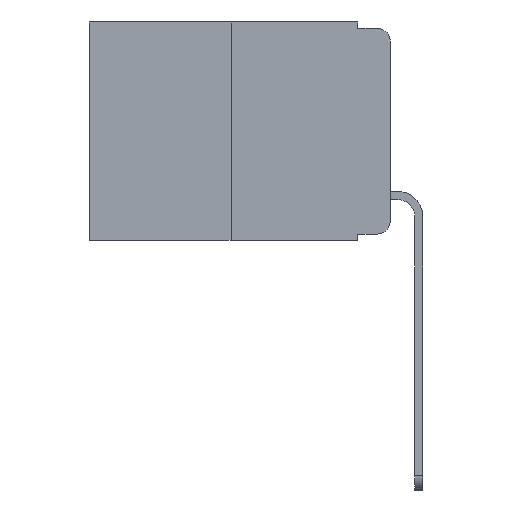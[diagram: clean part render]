
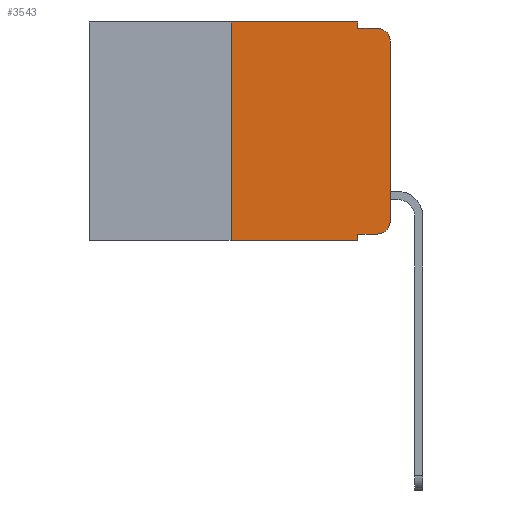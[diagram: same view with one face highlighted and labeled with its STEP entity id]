
A CAD part, left-side view. The second image highlights one B-rep face of the part: STEP entity #3543.
In plain terms, the highlighted planar face has unit normal (-1, 0, 0).
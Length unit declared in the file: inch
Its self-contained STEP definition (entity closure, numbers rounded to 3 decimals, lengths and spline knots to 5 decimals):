
#118 = VECTOR ( 'NONE', #10049, 39.37008 ) ;
#206 = EDGE_CURVE ( 'NONE', #10461, #6920, #1319, .T. ) ;
#211 = ORIENTED_EDGE ( 'NONE', *, *, #8891, .F. ) ;
#290 = DIRECTION ( 'NONE',  ( 0., 0., -1. ) ) ;
#351 = AXIS2_PLACEMENT_3D ( 'NONE', #6485, #12256, #6536 ) ;
#1319 = LINE ( 'NONE', #1860, #9890 ) ;
#1368 = DIRECTION ( 'NONE',  ( 0., 0., -1. ) ) ;
#1842 = CARTESIAN_POINT ( 'NONE',  ( 0., 0., -0.03 ) ) ;
#1860 = CARTESIAN_POINT ( 'NONE',  ( 0., 0.473, 0. ) ) ;
#2236 = LINE ( 'NONE', #7683, #118 ) ;
#2592 = CARTESIAN_POINT ( 'NONE',  ( 0., 0., -0.313 ) ) ;
#2613 = CARTESIAN_POINT ( 'NONE',  ( 0., 0.02, -0.01 ) ) ;
#2663 = DIRECTION ( 'NONE',  ( 0., -1., 0. ) ) ;
#2763 = CARTESIAN_POINT ( 'NONE',  ( 0., 0.051, -0.01 ) ) ;
#3039 = DIRECTION ( 'NONE',  ( 0., 0., -1. ) ) ;
#3083 = CARTESIAN_POINT ( 'NONE',  ( 0., 0.051, -0.333 ) ) ;
#3187 = ORIENTED_EDGE ( 'NONE', *, *, #206, .F. ) ;
#3426 = VERTEX_POINT ( 'NONE', #9632 ) ;
#3506 = CIRCLE ( 'NONE', #7807, 0.02 ) ;
#3536 = LINE ( 'NONE', #11084, #14057 ) ;
#3543 = ADVANCED_FACE ( 'NONE', ( #4294 ), #5477, .F. ) ;
#3706 = EDGE_CURVE ( 'NONE', #3426, #8450, #5513, .T. ) ;
#4294 = FACE_OUTER_BOUND ( 'NONE', #13301, .T. ) ;
#4432 = VECTOR ( 'NONE', #2663, 39.37008 ) ;
#4646 = CARTESIAN_POINT ( 'NONE',  ( 0., 0.051, 0. ) ) ;
#4722 = EDGE_CURVE ( 'NONE', #13877, #8409, #13920, .T. ) ;
#4989 = CARTESIAN_POINT ( 'NONE',  ( 0., 0.25, 0. ) ) ;
#5438 = LINE ( 'NONE', #4646, #9272 ) ;
#5477 = PLANE ( 'NONE',  #351 ) ;
#5513 = CIRCLE ( 'NONE', #7577, 0.02 ) ;
#5728 = LINE ( 'NONE', #8766, #8322 ) ;
#5772 = ORIENTED_EDGE ( 'NONE', *, *, #9469, .T. ) ;
#5774 = VECTOR ( 'NONE', #11662, 39.37008 ) ;
#5886 = CARTESIAN_POINT ( 'NONE',  ( 0., 0.02, -0.03 ) ) ;
#6485 = CARTESIAN_POINT ( 'NONE',  ( 0., 0.473, 0. ) ) ;
#6527 = VERTEX_POINT ( 'NONE', #2613 ) ;
#6536 = DIRECTION ( 'NONE',  ( 0., 0., -1. ) ) ;
#6716 = DIRECTION ( 'NONE',  ( 0., -1., 0. ) ) ;
#6920 = VERTEX_POINT ( 'NONE', #13278 ) ;
#6983 = ORIENTED_EDGE ( 'NONE', *, *, #3706, .T. ) ;
#7577 = AXIS2_PLACEMENT_3D ( 'NONE', #10652, #14409, #3039 ) ;
#7683 = CARTESIAN_POINT ( 'NONE',  ( 0., 0.051, -0.01 ) ) ;
#7807 = AXIS2_PLACEMENT_3D ( 'NONE', #5886, #13757, #290 ) ;
#7936 = CARTESIAN_POINT ( 'NONE',  ( 0., 0., 0. ) ) ;
#8148 = CARTESIAN_POINT ( 'NONE',  ( 0., 0.051, -0.343 ) ) ;
#8176 = VERTEX_POINT ( 'NONE', #3083 ) ;
#8322 = VECTOR ( 'NONE', #8817, 39.37008 ) ;
#8409 = VERTEX_POINT ( 'NONE', #8148 ) ;
#8450 = VERTEX_POINT ( 'NONE', #2592 ) ;
#8682 = CARTESIAN_POINT ( 'NONE',  ( 0., 0.25, 0. ) ) ;
#8766 = CARTESIAN_POINT ( 'NONE',  ( 0., 0.051, 0. ) ) ;
#8817 = DIRECTION ( 'NONE',  ( 0., 0., -1. ) ) ;
#8891 = EDGE_CURVE ( 'NONE', #6920, #11487, #5728, .T. ) ;
#9255 = CARTESIAN_POINT ( 'NONE',  ( 0., 0.473, -0.343 ) ) ;
#9272 = VECTOR ( 'NONE', #1368, 39.37008 ) ;
#9469 = EDGE_CURVE ( 'NONE', #8450, #10483, #13219, .T. ) ;
#9632 = CARTESIAN_POINT ( 'NONE',  ( 0., 0.02, -0.333 ) ) ;
#9890 = VECTOR ( 'NONE', #11973, 39.37008 ) ;
#9995 = DIRECTION ( 'NONE',  ( 0., 0., 1. ) ) ;
#10049 = DIRECTION ( 'NONE',  ( 0., -1., 0. ) ) ;
#10373 = CARTESIAN_POINT ( 'NONE',  ( 0., 0.25, -0.343 ) ) ;
#10461 = VERTEX_POINT ( 'NONE', #8682 ) ;
#10483 = VERTEX_POINT ( 'NONE', #1842 ) ;
#10493 = ORIENTED_EDGE ( 'NONE', *, *, #11947, .T. ) ;
#10652 = CARTESIAN_POINT ( 'NONE',  ( 0., 0.02, -0.313 ) ) ;
#10686 = EDGE_CURVE ( 'NONE', #8176, #8409, #5438, .T. ) ;
#11084 = CARTESIAN_POINT ( 'NONE',  ( 0., 0.051, -0.333 ) ) ;
#11184 = ORIENTED_EDGE ( 'NONE', *, *, #12038, .F. ) ;
#11224 = EDGE_CURVE ( 'NONE', #8176, #3426, #3536, .T. ) ;
#11487 = VERTEX_POINT ( 'NONE', #2763 ) ;
#11662 = DIRECTION ( 'NONE',  ( 0., 0., 1. ) ) ;
#11689 = ORIENTED_EDGE ( 'NONE', *, *, #10686, .F. ) ;
#11947 = EDGE_CURVE ( 'NONE', #10483, #6527, #3506, .T. ) ;
#11973 = DIRECTION ( 'NONE',  ( 0., -1., 0. ) ) ;
#12038 = EDGE_CURVE ( 'NONE', #13877, #10461, #12462, .T. ) ;
#12256 = DIRECTION ( 'NONE',  ( 1., 0., 0. ) ) ;
#12462 = LINE ( 'NONE', #4989, #5774 ) ;
#12803 = ORIENTED_EDGE ( 'NONE', *, *, #11224, .T. ) ;
#12995 = EDGE_CURVE ( 'NONE', #11487, #6527, #2236, .T. ) ;
#13127 = ORIENTED_EDGE ( 'NONE', *, *, #12995, .F. ) ;
#13219 = LINE ( 'NONE', #7936, #13398 ) ;
#13278 = CARTESIAN_POINT ( 'NONE',  ( 0., 0.051, 0. ) ) ;
#13301 = EDGE_LOOP ( 'NONE', ( #5772, #10493, #13127, #211, #3187, #11184, #13602, #11689, #12803, #6983 ) ) ;
#13398 = VECTOR ( 'NONE', #9995, 39.37008 ) ;
#13602 = ORIENTED_EDGE ( 'NONE', *, *, #4722, .T. ) ;
#13757 = DIRECTION ( 'NONE',  ( -1., 0., 0. ) ) ;
#13877 = VERTEX_POINT ( 'NONE', #10373 ) ;
#13920 = LINE ( 'NONE', #9255, #4432 ) ;
#14057 = VECTOR ( 'NONE', #6716, 39.37008 ) ;
#14409 = DIRECTION ( 'NONE',  ( -1., 0., 0. ) ) ;
